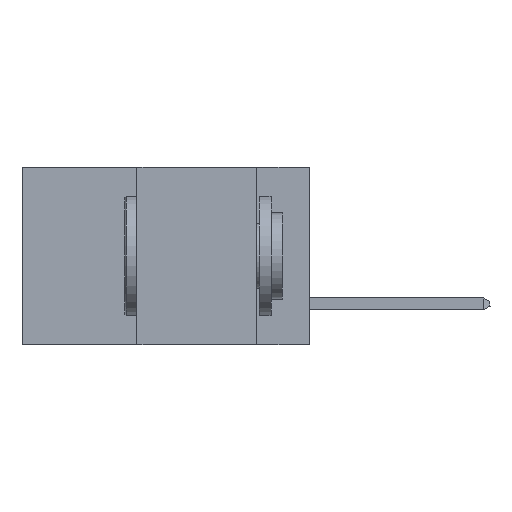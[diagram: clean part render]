
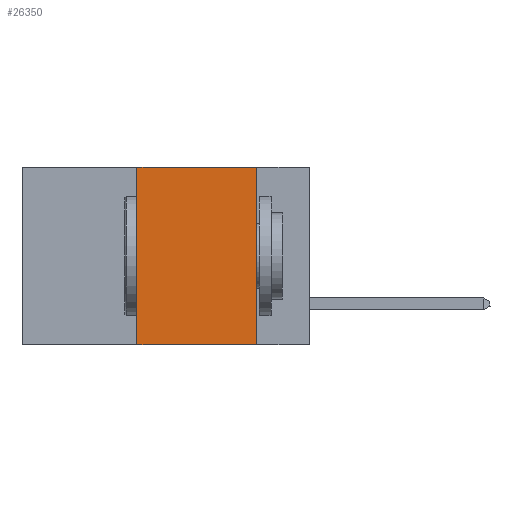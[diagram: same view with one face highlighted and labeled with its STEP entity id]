
A CAD part, left-side view. The second image highlights one B-rep face of the part: STEP entity #26350.
In plain terms, the highlighted planar face has unit normal (-1, 0, 0).
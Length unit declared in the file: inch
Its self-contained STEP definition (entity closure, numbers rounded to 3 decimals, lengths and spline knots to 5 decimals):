
#1217 = VECTOR ( 'NONE', #8665, 39.37008 ) ;
#4648 = DIRECTION ( 'NONE',  ( 0., -1., 0. ) ) ;
#4837 = LINE ( 'NONE', #13061, #15389 ) ;
#5977 = VERTEX_POINT ( 'NONE', #32050 ) ;
#8568 = VECTOR ( 'NONE', #4648, 39.37008 ) ;
#8665 = DIRECTION ( 'NONE',  ( 0., 0., -1. ) ) ;
#9067 = CARTESIAN_POINT ( 'NONE',  ( 0., 0.6, 0. ) ) ;
#11682 = EDGE_CURVE ( 'NONE', #32399, #31505, #13777, .T. ) ;
#12087 = DIRECTION ( 'NONE',  ( 1., 0., 0. ) ) ;
#12122 = ORIENTED_EDGE ( 'NONE', *, *, #17692, .F. ) ;
#12248 = DIRECTION ( 'NONE',  ( 0., -1., 0. ) ) ;
#12580 = CARTESIAN_POINT ( 'NONE',  ( 0., 0.36, 0. ) ) ;
#13061 = CARTESIAN_POINT ( 'NONE',  ( 0., 0.36, 0. ) ) ;
#13406 = EDGE_LOOP ( 'NONE', ( #28296, #16758, #12122, #26499 ) ) ;
#13777 = LINE ( 'NONE', #9067, #14186 ) ;
#14186 = VECTOR ( 'NONE', #12248, 39.37008 ) ;
#15177 = VERTEX_POINT ( 'NONE', #16720 ) ;
#15389 = VECTOR ( 'NONE', #31328, 39.37008 ) ;
#16278 = LINE ( 'NONE', #25580, #8568 ) ;
#16720 = CARTESIAN_POINT ( 'NONE',  ( 0., 0.11, -0.37 ) ) ;
#16758 = ORIENTED_EDGE ( 'NONE', *, *, #11682, .F. ) ;
#16949 = CARTESIAN_POINT ( 'NONE',  ( 0., 0.6, 0. ) ) ;
#17692 = EDGE_CURVE ( 'NONE', #5977, #32399, #4837, .T. ) ;
#22005 = LINE ( 'NONE', #31946, #1217 ) ;
#22033 = EDGE_CURVE ( 'NONE', #5977, #15177, #16278, .T. ) ;
#23645 = FACE_OUTER_BOUND ( 'NONE', #13406, .T. ) ;
#25177 = PLANE ( 'NONE',  #30315 ) ;
#25580 = CARTESIAN_POINT ( 'NONE',  ( 0., 0.6, -0.37 ) ) ;
#26350 = ADVANCED_FACE ( 'NONE', ( #23645 ), #25177, .F. ) ;
#26499 = ORIENTED_EDGE ( 'NONE', *, *, #22033, .T. ) ;
#28296 = ORIENTED_EDGE ( 'NONE', *, *, #32591, .F. ) ;
#28882 = CARTESIAN_POINT ( 'NONE',  ( 0., 0.11, 0. ) ) ;
#30254 = DIRECTION ( 'NONE',  ( 0., 0., -1. ) ) ;
#30315 = AXIS2_PLACEMENT_3D ( 'NONE', #16949, #12087, #30254 ) ;
#31328 = DIRECTION ( 'NONE',  ( 0., 0., 1. ) ) ;
#31505 = VERTEX_POINT ( 'NONE', #28882 ) ;
#31946 = CARTESIAN_POINT ( 'NONE',  ( 0., 0.11, 0. ) ) ;
#32050 = CARTESIAN_POINT ( 'NONE',  ( 0., 0.36, -0.37 ) ) ;
#32399 = VERTEX_POINT ( 'NONE', #12580 ) ;
#32591 = EDGE_CURVE ( 'NONE', #31505, #15177, #22005, .T. ) ;
